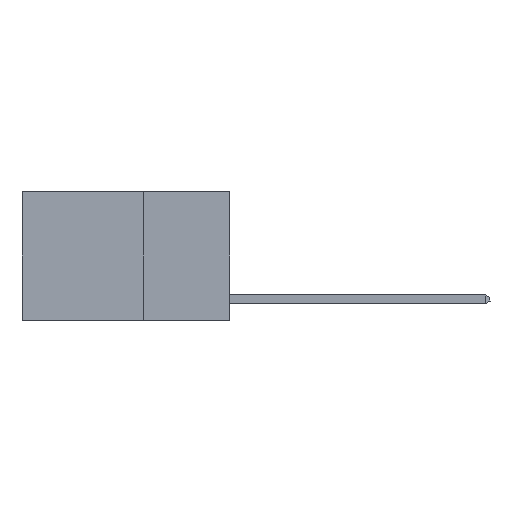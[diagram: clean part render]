
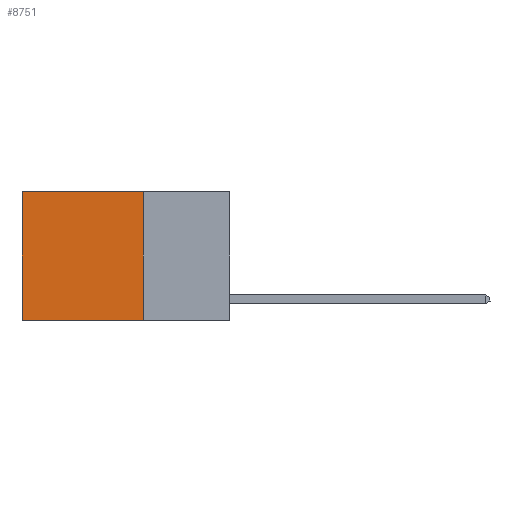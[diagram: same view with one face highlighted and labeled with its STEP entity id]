
A CAD part, left-side view. The second image highlights one B-rep face of the part: STEP entity #8751.
In plain terms, the highlighted planar face has unit normal (-1, 0, 0).
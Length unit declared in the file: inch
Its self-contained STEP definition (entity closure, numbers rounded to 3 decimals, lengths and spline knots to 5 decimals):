
#251 = VERTEX_POINT ( 'NONE', #2044 ) ;
#2008 = FACE_OUTER_BOUND ( 'NONE', #18739, .T. ) ;
#2044 = CARTESIAN_POINT ( 'NONE',  ( 0.2625, 0.6, 0. ) ) ;
#2122 = LINE ( 'NONE', #17859, #13696 ) ;
#4016 = VECTOR ( 'NONE', #7946, 39.37008 ) ;
#4543 = CARTESIAN_POINT ( 'NONE',  ( 0.2625, 0.6, -0.37 ) ) ;
#5278 = ORIENTED_EDGE ( 'NONE', *, *, #14190, .T. ) ;
#5577 = AXIS2_PLACEMENT_3D ( 'NONE', #17839, #6362, #15084 ) ;
#5746 = EDGE_CURVE ( 'NONE', #9527, #6843, #16757, .T. ) ;
#6362 = DIRECTION ( 'NONE',  ( 1., 0., 0. ) ) ;
#6843 = VERTEX_POINT ( 'NONE', #15140 ) ;
#7042 = VECTOR ( 'NONE', #10219, 39.37008 ) ;
#7699 = PLANE ( 'NONE',  #5577 ) ;
#7946 = DIRECTION ( 'NONE',  ( 0., 1., 0. ) ) ;
#8751 = ADVANCED_FACE ( 'NONE', ( #2008 ), #7699, .F. ) ;
#9527 = VERTEX_POINT ( 'NONE', #18139 ) ;
#9722 = DIRECTION ( 'NONE',  ( 0., 0., -1. ) ) ;
#10114 = VECTOR ( 'NONE', #9722, 39.37008 ) ;
#10219 = DIRECTION ( 'NONE',  ( 0., 1., 0. ) ) ;
#10703 = LINE ( 'NONE', #14013, #4016 ) ;
#11631 = VERTEX_POINT ( 'NONE', #4543 ) ;
#12049 = ORIENTED_EDGE ( 'NONE', *, *, #14624, .T. ) ;
#12516 = ORIENTED_EDGE ( 'NONE', *, *, #5746, .F. ) ;
#13240 = LINE ( 'NONE', #14863, #7042 ) ;
#13696 = VECTOR ( 'NONE', #18046, 39.37008 ) ;
#13851 = EDGE_CURVE ( 'NONE', #6843, #11631, #10703, .T. ) ;
#14013 = CARTESIAN_POINT ( 'NONE',  ( 0.2625, 0.25, -0.37 ) ) ;
#14190 = EDGE_CURVE ( 'NONE', #9527, #251, #13240, .T. ) ;
#14624 = EDGE_CURVE ( 'NONE', #251, #11631, #2122, .T. ) ;
#14863 = CARTESIAN_POINT ( 'NONE',  ( 0.2625, 0.25, 0. ) ) ;
#15084 = DIRECTION ( 'NONE',  ( 0., 0., -1. ) ) ;
#15140 = CARTESIAN_POINT ( 'NONE',  ( 0.2625, 0.25, -0.37 ) ) ;
#15423 = ORIENTED_EDGE ( 'NONE', *, *, #13851, .F. ) ;
#16658 = CARTESIAN_POINT ( 'NONE',  ( 0.2625, 0.25, 0. ) ) ;
#16757 = LINE ( 'NONE', #16658, #10114 ) ;
#17839 = CARTESIAN_POINT ( 'NONE',  ( 0.2625, 0.25, 0. ) ) ;
#17859 = CARTESIAN_POINT ( 'NONE',  ( 0.2625, 0.6, 0. ) ) ;
#18046 = DIRECTION ( 'NONE',  ( 0., 0., -1. ) ) ;
#18139 = CARTESIAN_POINT ( 'NONE',  ( 0.2625, 0.25, 0. ) ) ;
#18739 = EDGE_LOOP ( 'NONE', ( #12049, #15423, #12516, #5278 ) ) ;
